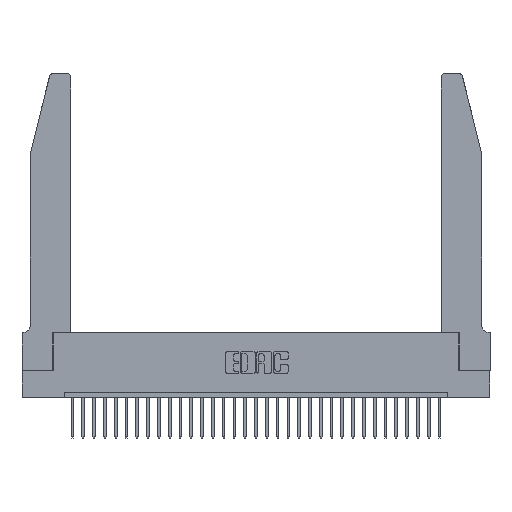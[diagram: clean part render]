
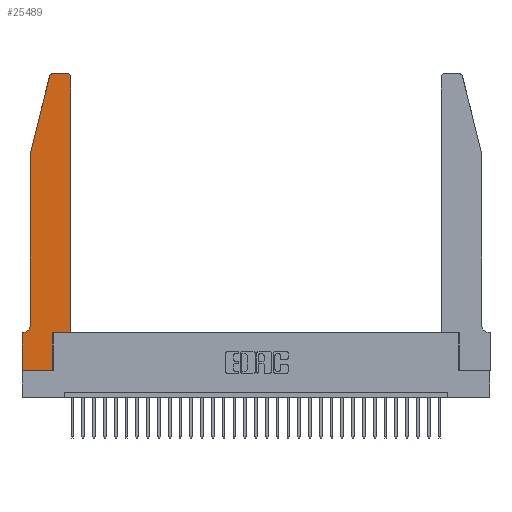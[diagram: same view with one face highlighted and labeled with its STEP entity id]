
A CAD part, top view. The second image highlights one B-rep face of the part: STEP entity #25489.
In plain terms, the highlighted planar face has unit normal (0, 0, 1).
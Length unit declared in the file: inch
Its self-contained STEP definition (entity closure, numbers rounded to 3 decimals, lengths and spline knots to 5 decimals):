
#128 = LINE ( 'NONE', #31623, #24948 ) ;
#566 = DIRECTION ( 'NONE',  ( 0., 0., 1. ) ) ;
#1259 = DIRECTION ( 'NONE',  ( 0., -1., 0. ) ) ;
#1428 = PLANE ( 'NONE',  #16719 ) ;
#1681 = CARTESIAN_POINT ( 'NONE',  ( 0.284, 2.75, 0.37 ) ) ;
#1795 = EDGE_CURVE ( 'NONE', #3997, #3652, #5463, .T. ) ;
#1831 = DIRECTION ( 'NONE',  ( 1., 0., 0. ) ) ;
#2629 = CARTESIAN_POINT ( 'NONE',  ( 0.2865, 0., 0.37 ) ) ;
#3408 = LINE ( 'NONE', #9713, #31301 ) ;
#3652 = VERTEX_POINT ( 'NONE', #19888 ) ;
#3751 = EDGE_CURVE ( 'NONE', #3652, #25780, #3408, .T. ) ;
#3997 = VERTEX_POINT ( 'NONE', #2629 ) ;
#4235 = CARTESIAN_POINT ( 'NONE',  ( 0.0755, 0.35, 0.37 ) ) ;
#4375 = EDGE_CURVE ( 'NONE', #18408, #9417, #16978, .T. ) ;
#5463 = LINE ( 'NONE', #6913, #9367 ) ;
#5832 = ORIENTED_EDGE ( 'NONE', *, *, #11748, .T. ) ;
#6097 = VECTOR ( 'NONE', #18073, 39.37008 ) ;
#6176 = DIRECTION ( 'NONE',  ( 0., 1., 0. ) ) ;
#6800 = ORIENTED_EDGE ( 'NONE', *, *, #19224, .T. ) ;
#6913 = CARTESIAN_POINT ( 'NONE',  ( 0.2865, 0.35, 0.37 ) ) ;
#7149 = DIRECTION ( 'NONE',  ( 1., 0., 0. ) ) ;
#7360 = VECTOR ( 'NONE', #11507, 39.37008 ) ;
#8552 = DIRECTION ( 'NONE',  ( 0., 0., -1. ) ) ;
#8918 = EDGE_CURVE ( 'NONE', #25780, #28432, #29999, .T. ) ;
#9345 = CARTESIAN_POINT ( 'NONE',  ( 0., 0., 0.37 ) ) ;
#9367 = VECTOR ( 'NONE', #11941, 39.37008 ) ;
#9417 = VERTEX_POINT ( 'NONE', #1681 ) ;
#9640 = DIRECTION ( 'NONE',  ( -1., 0., 0. ) ) ;
#9713 = CARTESIAN_POINT ( 'NONE',  ( 0.4505, 0.35, 0.37 ) ) ;
#10644 = CARTESIAN_POINT ( 'NONE',  ( 0.284, 2.72, 0.37 ) ) ;
#11081 = CARTESIAN_POINT ( 'NONE',  ( 0.0055, 0.42, 0.37 ) ) ;
#11186 = ORIENTED_EDGE ( 'NONE', *, *, #1795, .T. ) ;
#11507 = DIRECTION ( 'NONE',  ( -1., 0., 0. ) ) ;
#11680 = VECTOR ( 'NONE', #14723, 39.37008 ) ;
#11748 = EDGE_CURVE ( 'NONE', #19816, #28822, #27177, .T. ) ;
#11941 = DIRECTION ( 'NONE',  ( 0., 1., 0. ) ) ;
#13682 = DIRECTION ( 'NONE',  ( 1., 0., 0. ) ) ;
#14108 = CARTESIAN_POINT ( 'NONE',  ( 0.4505, 2.72, 0.37 ) ) ;
#14230 = AXIS2_PLACEMENT_3D ( 'NONE', #10644, #566, #15056 ) ;
#14276 = VERTEX_POINT ( 'NONE', #9345 ) ;
#14693 = EDGE_CURVE ( 'NONE', #9417, #24601, #30116, .T. ) ;
#14723 = DIRECTION ( 'NONE',  ( 0., -1., 0. ) ) ;
#15056 = DIRECTION ( 'NONE',  ( 1., 0., 0. ) ) ;
#15392 = VECTOR ( 'NONE', #9640, 39.37008 ) ;
#15648 = CARTESIAN_POINT ( 'NONE',  ( 0.4505, 0.35, 0.37 ) ) ;
#16648 = ORIENTED_EDGE ( 'NONE', *, *, #21549, .T. ) ;
#16719 = AXIS2_PLACEMENT_3D ( 'NONE', #21330, #18459, #13682 ) ;
#16978 = LINE ( 'NONE', #22000, #15392 ) ;
#17007 = LINE ( 'NONE', #17843, #6097 ) ;
#17843 = CARTESIAN_POINT ( 'NONE',  ( 0.0755, 2., 0.37 ) ) ;
#18073 = DIRECTION ( 'NONE',  ( -0.239, -0.971, 0. ) ) ;
#18188 = EDGE_CURVE ( 'NONE', #28822, #18371, #30648, .T. ) ;
#18216 = CARTESIAN_POINT ( 'NONE',  ( 0.0755, 0.42, 0.37 ) ) ;
#18257 = LINE ( 'NONE', #4235, #7360 ) ;
#18273 = LINE ( 'NONE', #25103, #11680 ) ;
#18290 = CARTESIAN_POINT ( 'NONE',  ( 0.0755, 2., 0.37 ) ) ;
#18371 = VERTEX_POINT ( 'NONE', #20075 ) ;
#18408 = VERTEX_POINT ( 'NONE', #25830 ) ;
#18459 = DIRECTION ( 'NONE',  ( 0., 0., 1. ) ) ;
#18573 = CARTESIAN_POINT ( 'NONE',  ( 0.4505, 0.35, 0.37 ) ) ;
#18901 = ORIENTED_EDGE ( 'NONE', *, *, #4375, .T. ) ;
#19224 = EDGE_CURVE ( 'NONE', #28432, #18408, #23724, .T. ) ;
#19454 = VECTOR ( 'NONE', #1259, 39.37008 ) ;
#19816 = VERTEX_POINT ( 'NONE', #29444 ) ;
#19888 = CARTESIAN_POINT ( 'NONE',  ( 0.2865, 0.35, 0.37 ) ) ;
#20075 = CARTESIAN_POINT ( 'NONE',  ( 0.0055, 0.35, 0.37 ) ) ;
#20293 = EDGE_CURVE ( 'NONE', #31435, #14276, #18273, .T. ) ;
#21330 = CARTESIAN_POINT ( 'NONE',  ( 0., 0.35, 0.37 ) ) ;
#21549 = EDGE_CURVE ( 'NONE', #24601, #19816, #17007, .T. ) ;
#21581 = ORIENTED_EDGE ( 'NONE', *, *, #3751, .T. ) ;
#22000 = CARTESIAN_POINT ( 'NONE',  ( 0.2605, 2.75, 0.37 ) ) ;
#22361 = AXIS2_PLACEMENT_3D ( 'NONE', #11081, #8552, #23199 ) ;
#23143 = ORIENTED_EDGE ( 'NONE', *, *, #18188, .T. ) ;
#23199 = DIRECTION ( 'NONE',  ( -1., 0., 0. ) ) ;
#23724 = CIRCLE ( 'NONE', #30010, 0.03 ) ;
#23817 = DIRECTION ( 'NONE',  ( 1., 0., 0. ) ) ;
#24033 = DIRECTION ( 'NONE',  ( 0., 0., 1. ) ) ;
#24601 = VERTEX_POINT ( 'NONE', #24713 ) ;
#24713 = CARTESIAN_POINT ( 'NONE',  ( 0.25487, 2.72718, 0.37 ) ) ;
#24716 = CARTESIAN_POINT ( 'NONE',  ( 0., 0.35, 0.37 ) ) ;
#24932 = EDGE_CURVE ( 'NONE', #14276, #3997, #128, .T. ) ;
#24948 = VECTOR ( 'NONE', #7149, 39.37008 ) ;
#25103 = CARTESIAN_POINT ( 'NONE',  ( 0., 0., 0.37 ) ) ;
#25263 = FACE_OUTER_BOUND ( 'NONE', #26507, .T. ) ;
#25489 = ADVANCED_FACE ( 'NONE', ( #25263 ), #1428, .T. ) ;
#25500 = ORIENTED_EDGE ( 'NONE', *, *, #20293, .T. ) ;
#25780 = VERTEX_POINT ( 'NONE', #15648 ) ;
#25830 = CARTESIAN_POINT ( 'NONE',  ( 0.4205, 2.75, 0.37 ) ) ;
#25851 = ORIENTED_EDGE ( 'NONE', *, *, #24932, .T. ) ;
#26071 = CARTESIAN_POINT ( 'NONE',  ( 0.4205, 2.72, 0.37 ) ) ;
#26507 = EDGE_LOOP ( 'NONE', ( #18901, #29854, #16648, #5832, #23143, #31224, #25500, #25851, #11186, #21581, #31459, #6800 ) ) ;
#27177 = LINE ( 'NONE', #18290, #19454 ) ;
#28432 = VERTEX_POINT ( 'NONE', #14108 ) ;
#28822 = VERTEX_POINT ( 'NONE', #18216 ) ;
#29444 = CARTESIAN_POINT ( 'NONE',  ( 0.0755, 2., 0.37 ) ) ;
#29854 = ORIENTED_EDGE ( 'NONE', *, *, #14693, .T. ) ;
#29999 = LINE ( 'NONE', #18573, #31935 ) ;
#30010 = AXIS2_PLACEMENT_3D ( 'NONE', #26071, #24033, #23817 ) ;
#30116 = CIRCLE ( 'NONE', #14230, 0.03 ) ;
#30648 = CIRCLE ( 'NONE', #22361, 0.07 ) ;
#31183 = EDGE_CURVE ( 'NONE', #18371, #31435, #18257, .T. ) ;
#31224 = ORIENTED_EDGE ( 'NONE', *, *, #31183, .T. ) ;
#31301 = VECTOR ( 'NONE', #1831, 39.37008 ) ;
#31435 = VERTEX_POINT ( 'NONE', #24716 ) ;
#31459 = ORIENTED_EDGE ( 'NONE', *, *, #8918, .T. ) ;
#31623 = CARTESIAN_POINT ( 'NONE',  ( 0., 0., 0.37 ) ) ;
#31935 = VECTOR ( 'NONE', #6176, 39.37008 ) ;
